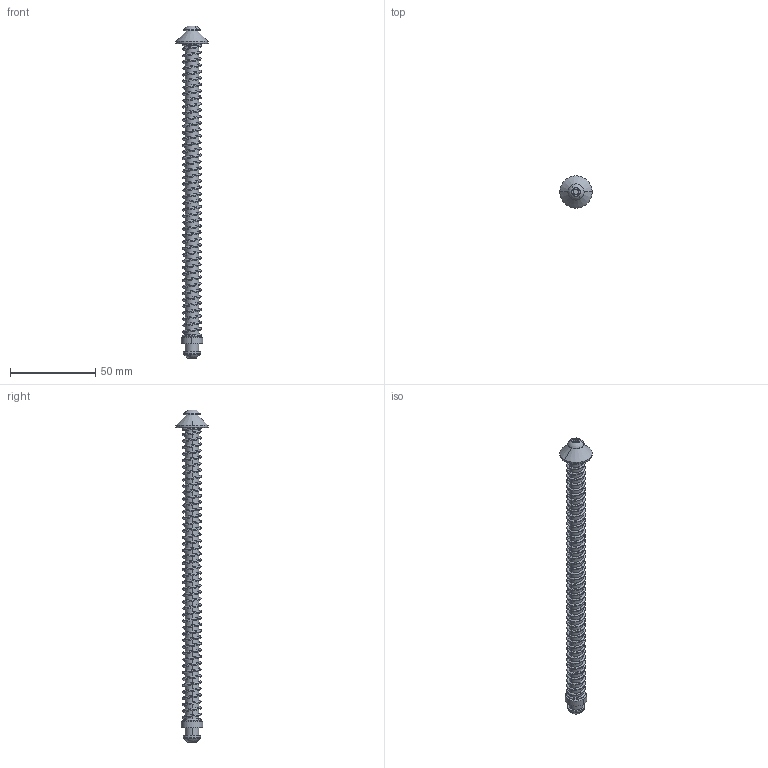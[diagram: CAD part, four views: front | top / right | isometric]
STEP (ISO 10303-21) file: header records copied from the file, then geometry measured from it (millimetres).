
FILE_DESCRIPTION (( 'STEP AP214' ), '1' );
FILE_NAME ('PPDW9 V4 Recoil rod and spring.STEP', '2020-12-31T18:26:07', ( '' ), ( '' ), 'SwSTEP 2.0', 'SolidWorks 2020', '' );
FILE_SCHEMA (( 'AUTOMOTIVE_DESIGN' ));
Length unit declared in the file: inch
Products named in the file (8): M5 x 12mm BHSH 91239A228_BLACK_91239A228; PPDW9 V4  AK47 Recoil Spring cut to 8in_94125K22; M5 x 16mm BHSHCS 91239A232_91239A232; PPDW9 V2 - V4 Recoil rod end; M5 flat washer 98269A440_BLACK_98269A440; recoil rod stop HK UMP; PPDW9 V4  Recoil rod; PPDW9 V4 Recoil rod and spring
Assembly tree (7 placements, depth 2):
  PPDW9 V4 Recoil rod and spring
    PPDW9 V4  Recoil rod
    PPDW9 V4  AK47 Recoil Spring cut to 8in_94125K22
    recoil rod stop HK UMP
    PPDW9 V2 - V4 Recoil rod end
    M5 x 16mm BHSHCS 91239A232_91239A232
    M5 flat washer 98269A440_BLACK_98269A440
    M5 x 12mm BHSH 91239A228_BLACK_91239A228
Bounding box: 19 x 19 x 195.19 mm (x, y, z)
Volume: 12753.9 mm3; surface area: 13295 mm2
Topology: 7 solids, 7 shells, 238 faces, 617 edges, 395 vertices
Faces by surface type: cylinder 162, plane 32, cone 26, bspline 10, torus 4, sphere 4
Entity records: 20888 total; most frequent: CARTESIAN_POINT 15546, ORIENTED_EDGE 1226, DIRECTION 864, EDGE_CURVE 613, VERTEX_POINT 395, AXIS2_PLACEMENT_3D 333, EDGE_LOOP 250, FACE_OUTER_BOUND 238
